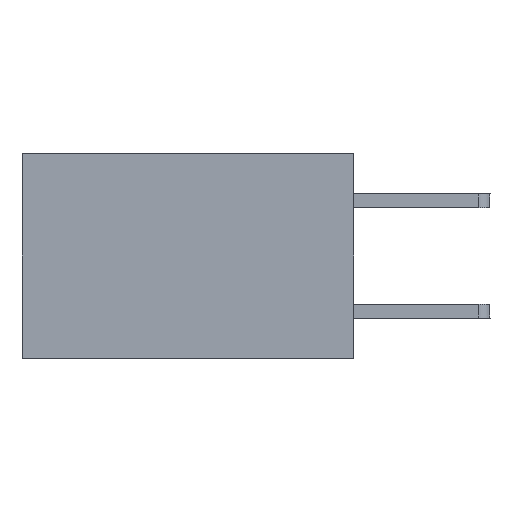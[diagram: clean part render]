
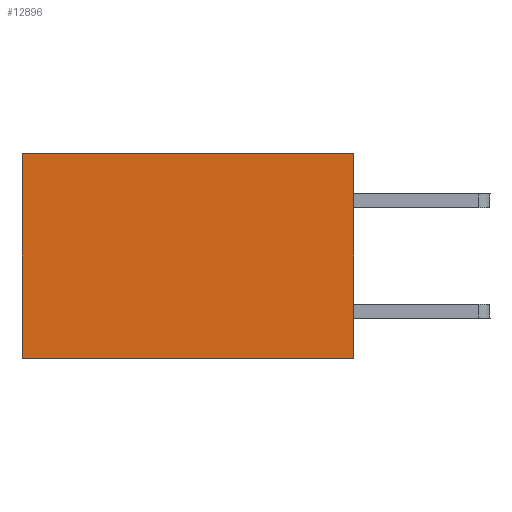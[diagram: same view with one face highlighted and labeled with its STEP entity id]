
A CAD part, left-side view. The second image highlights one B-rep face of the part: STEP entity #12896.
In plain terms, the highlighted planar face has unit normal (-1, 0, 0).
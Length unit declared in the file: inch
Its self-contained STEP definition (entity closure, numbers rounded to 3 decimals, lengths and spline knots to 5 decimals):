
#547 = PLANE ( 'NONE',  #13031 ) ;
#693 = VERTEX_POINT ( 'NONE', #16430 ) ;
#716 = DIRECTION ( 'NONE',  ( 1., 0., 0. ) ) ;
#856 = VECTOR ( 'NONE', #3958, 39.37008 ) ;
#1273 = LINE ( 'NONE', #9388, #856 ) ;
#1698 = VERTEX_POINT ( 'NONE', #5895 ) ;
#2278 = DIRECTION ( 'NONE',  ( 0., 1., 0. ) ) ;
#2410 = VECTOR ( 'NONE', #7317, 39.37008 ) ;
#2826 = EDGE_CURVE ( 'NONE', #13013, #693, #1273, .T. ) ;
#3958 = DIRECTION ( 'NONE',  ( 0., 0., -1. ) ) ;
#4398 = FACE_OUTER_BOUND ( 'NONE', #6059, .T. ) ;
#4670 = LINE ( 'NONE', #12650, #8147 ) ;
#5258 = VECTOR ( 'NONE', #13939, 39.37008 ) ;
#5895 = CARTESIAN_POINT ( 'NONE',  ( 0.2875, 0.6, 0. ) ) ;
#6059 = EDGE_LOOP ( 'NONE', ( #16609, #16379, #7824, #13957 ) ) ;
#6218 = VERTEX_POINT ( 'NONE', #8898 ) ;
#6286 = EDGE_CURVE ( 'NONE', #13013, #1698, #4670, .T. ) ;
#7096 = EDGE_CURVE ( 'NONE', #1698, #6218, #13074, .T. ) ;
#7236 = CARTESIAN_POINT ( 'NONE',  ( 0.2875, 0., 0. ) ) ;
#7317 = DIRECTION ( 'NONE',  ( 0., 1., 0. ) ) ;
#7608 = CARTESIAN_POINT ( 'NONE',  ( 0.2875, 0.6, 0. ) ) ;
#7824 = ORIENTED_EDGE ( 'NONE', *, *, #2826, .F. ) ;
#8147 = VECTOR ( 'NONE', #2278, 39.37008 ) ;
#8898 = CARTESIAN_POINT ( 'NONE',  ( 0.2875, 0.6, -0.37 ) ) ;
#9359 = LINE ( 'NONE', #14868, #2410 ) ;
#9388 = CARTESIAN_POINT ( 'NONE',  ( 0.2875, 0., 0. ) ) ;
#9701 = DIRECTION ( 'NONE',  ( 0., 0., -1. ) ) ;
#11157 = EDGE_CURVE ( 'NONE', #693, #6218, #9359, .T. ) ;
#12650 = CARTESIAN_POINT ( 'NONE',  ( 0.2875, 0., 0. ) ) ;
#12896 = ADVANCED_FACE ( 'NONE', ( #4398 ), #547, .F. ) ;
#13013 = VERTEX_POINT ( 'NONE', #13851 ) ;
#13031 = AXIS2_PLACEMENT_3D ( 'NONE', #7236, #716, #9701 ) ;
#13074 = LINE ( 'NONE', #7608, #5258 ) ;
#13851 = CARTESIAN_POINT ( 'NONE',  ( 0.2875, 0., 0. ) ) ;
#13939 = DIRECTION ( 'NONE',  ( 0., 0., -1. ) ) ;
#13957 = ORIENTED_EDGE ( 'NONE', *, *, #6286, .T. ) ;
#14868 = CARTESIAN_POINT ( 'NONE',  ( 0.2875, 0., -0.37 ) ) ;
#16379 = ORIENTED_EDGE ( 'NONE', *, *, #11157, .F. ) ;
#16430 = CARTESIAN_POINT ( 'NONE',  ( 0.2875, 0., -0.37 ) ) ;
#16609 = ORIENTED_EDGE ( 'NONE', *, *, #7096, .T. ) ;
